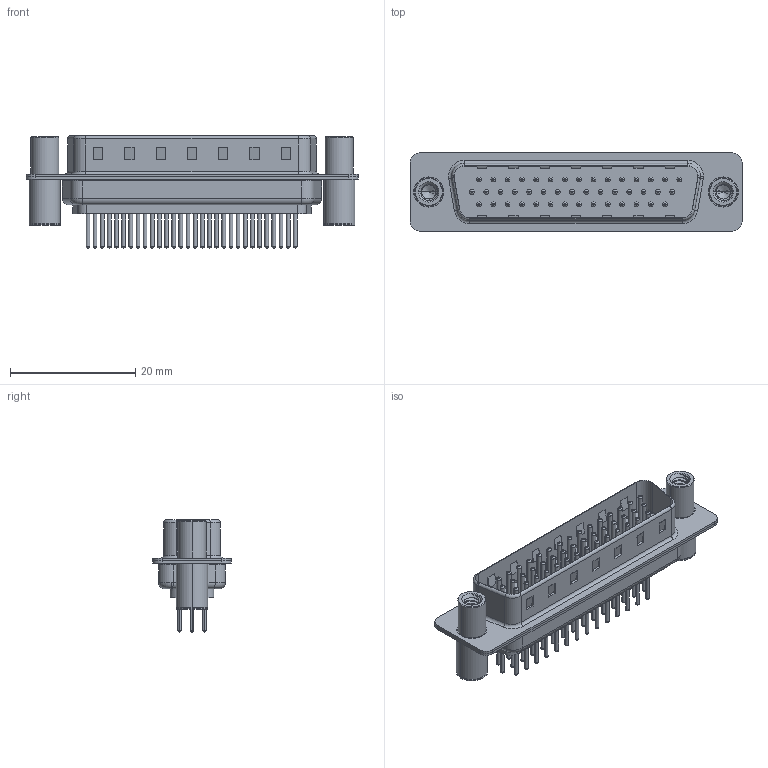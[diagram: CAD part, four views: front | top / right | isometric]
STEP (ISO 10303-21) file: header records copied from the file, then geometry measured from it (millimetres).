
FILE_DESCRIPTION (( 'STEP AP203' ), '1' );
FILE_NAME ('637-M44-630-BT4.STEP', '2018-11-20T01:38:21', ( '' ), ( '' ), 'SwSTEP 2.0', 'SolidWorks 2016', '' );
FILE_SCHEMA (( 'CONFIG_CONTROL_DESIGN' ));
Length unit declared in the file: millimetre
Products named in the file (8): 637M Shell Front_44 Contacts; 637M Shell Rear_44 Contacts; 637M Contact Row 1_30; 637M Contact Row 2_30; 637M Contact Row 3_30; 637M 4-40 Threaded Standoff and Board Spacer; 637-M44-630-BT4; 637M Housing_44 Contacts
Assembly tree (49 placements, depth 2):
  637-M44-630-BT4
    637M Housing_44 Contacts
    637M Shell Front_44 Contacts
    637M Shell Rear_44 Contacts
    637M Contact Row 1_30  x15
    637M Contact Row 2_30  x15
    637M Contact Row 3_30  x14
    637M 4-40 Threaded Standoff and Board Spacer  x2
Bounding box: 53.05 x 12.5 x 17.9 mm (x, y, z)
Volume: 3115.2 mm3; surface area: 8995.9 mm2
Topology: 49 solids, 49 shells, 2090 faces, 4439 edges, 2676 vertices
Faces by surface type: cylinder 805, torus 758, plane 485, cone 30, bspline 12
Entity records: 28385 total; most frequent: CARTESIAN_POINT 6363, DIRECTION 4566, ORIENTED_EDGE 3890, EDGE_CURVE 1945, AXIS2_PLACEMENT_3D 1850, VERTEX_POINT 1243, EDGE_LOOP 1062, CIRCLE 979
